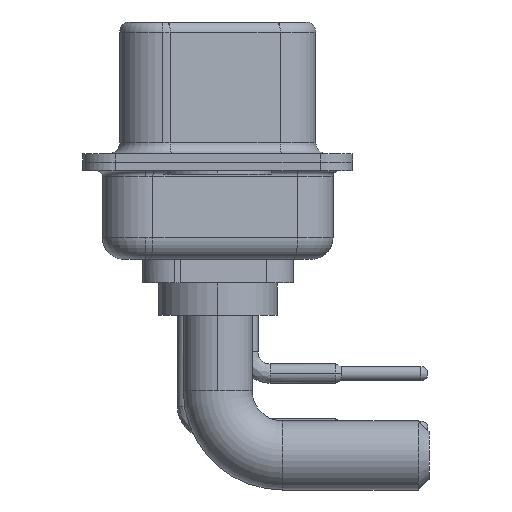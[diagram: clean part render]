
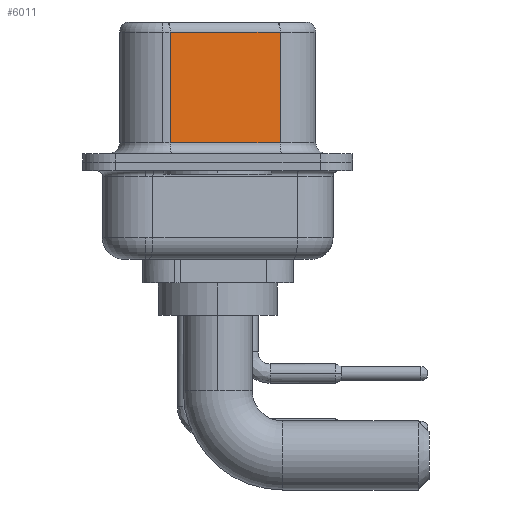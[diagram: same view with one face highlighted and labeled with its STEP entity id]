
A CAD part, left-side view. The second image highlights one B-rep face of the part: STEP entity #6011.
In plain terms, the highlighted planar face has unit normal (-0.985, -0.174, 0).
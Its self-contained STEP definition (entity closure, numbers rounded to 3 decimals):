
#446 = ORIENTED_EDGE ( 'NONE', *, *, #21582, .F. ) ;
#842 = CARTESIAN_POINT ( 'NONE',  ( 3.68, 2.203, 6.52 ) ) ;
#870 = AXIS2_PLACEMENT_3D ( 'NONE', #7345, #12961, #19506 ) ;
#1163 = EDGE_CURVE ( 'NONE', #1370, #7198, #3376, .T. ) ;
#1370 = VERTEX_POINT ( 'NONE', #19296 ) ;
#1474 = LINE ( 'NONE', #8363, #20771 ) ;
#2063 = FACE_OUTER_BOUND ( 'NONE', #8236, .T. ) ;
#3039 = DIRECTION ( 'NONE',  ( 0.174, -0.985, 0. ) ) ;
#3376 = LINE ( 'NONE', #18736, #5338 ) ;
#4301 = DIRECTION ( 'NONE',  ( 0., 0., -1. ) ) ;
#5338 = VECTOR ( 'NONE', #3039, 1000. ) ;
#6011 = ADVANCED_FACE ( 'NONE', ( #2063 ), #21334, .F. ) ;
#6341 = EDGE_CURVE ( 'NONE', #21532, #19329, #17520, .T. ) ;
#7198 = VERTEX_POINT ( 'NONE', #11990 ) ;
#7345 = CARTESIAN_POINT ( 'NONE',  ( 4.58, -2.897, 6.52 ) ) ;
#8088 = CARTESIAN_POINT ( 'NONE',  ( 3.68, 2.203, 6.02 ) ) ;
#8236 = EDGE_LOOP ( 'NONE', ( #446, #15926, #15220, #20544 ) ) ;
#8363 = CARTESIAN_POINT ( 'NONE',  ( 4.58, -2.897, 6.52 ) ) ;
#11990 = CARTESIAN_POINT ( 'NONE',  ( 4.58, -2.897, 0.9 ) ) ;
#12961 = DIRECTION ( 'NONE',  ( 0.985, 0.174, 0. ) ) ;
#13411 = VECTOR ( 'NONE', #4301, 1000. ) ;
#13990 = CARTESIAN_POINT ( 'NONE',  ( 4.58, -2.897, 6.02 ) ) ;
#14284 = VECTOR ( 'NONE', #22696, 1000. ) ;
#15220 = ORIENTED_EDGE ( 'NONE', *, *, #19422, .T. ) ;
#15362 = DIRECTION ( 'NONE',  ( 0., 0., -1. ) ) ;
#15926 = ORIENTED_EDGE ( 'NONE', *, *, #6341, .T. ) ;
#16452 = LINE ( 'NONE', #842, #13411 ) ;
#16844 = CARTESIAN_POINT ( 'NONE',  ( 4.58, -2.897, 6.02 ) ) ;
#17520 = LINE ( 'NONE', #13990, #14284 ) ;
#18736 = CARTESIAN_POINT ( 'NONE',  ( 4.58, -2.897, 0.9 ) ) ;
#19296 = CARTESIAN_POINT ( 'NONE',  ( 3.68, 2.203, 0.9 ) ) ;
#19329 = VERTEX_POINT ( 'NONE', #8088 ) ;
#19422 = EDGE_CURVE ( 'NONE', #19329, #1370, #16452, .T. ) ;
#19506 = DIRECTION ( 'NONE',  ( -0.174, 0.985, 0. ) ) ;
#20544 = ORIENTED_EDGE ( 'NONE', *, *, #1163, .T. ) ;
#20771 = VECTOR ( 'NONE', #15362, 1000. ) ;
#21334 = PLANE ( 'NONE',  #870 ) ;
#21532 = VERTEX_POINT ( 'NONE', #16844 ) ;
#21582 = EDGE_CURVE ( 'NONE', #21532, #7198, #1474, .T. ) ;
#22696 = DIRECTION ( 'NONE',  ( -0.174, 0.985, 0. ) ) ;
